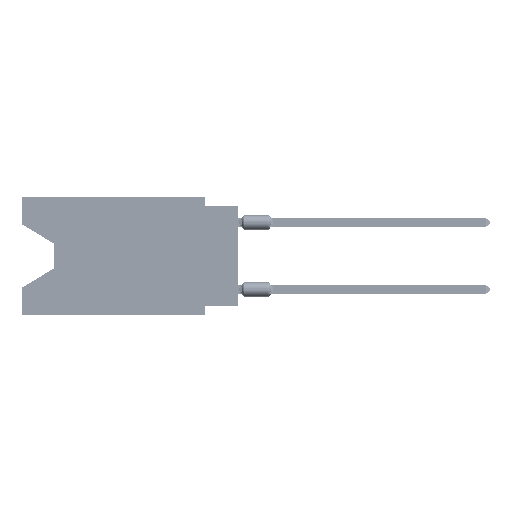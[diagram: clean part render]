
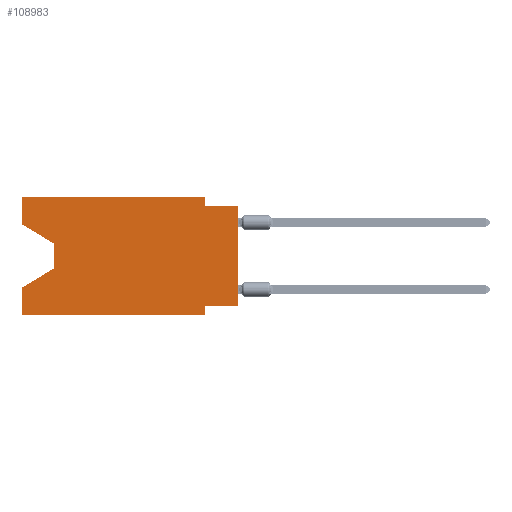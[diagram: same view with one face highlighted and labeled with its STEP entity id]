
A CAD part, left-side view. The second image highlights one B-rep face of the part: STEP entity #108983.
In plain terms, the highlighted planar face has unit normal (-1, 0, 0).
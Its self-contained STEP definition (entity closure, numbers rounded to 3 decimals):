
#1563 = LINE ( 'NONE', #73223, #68733 ) ;
#3938 = VECTOR ( 'NONE', #65482, 1000. ) ;
#7333 = EDGE_CURVE ( 'NONE', #61866, #8219, #95797, .T. ) ;
#8219 = VERTEX_POINT ( 'NONE', #72458 ) ;
#8479 = CARTESIAN_POINT ( 'NONE',  ( 0., 16.383, 0. ) ) ;
#8603 = EDGE_LOOP ( 'NONE', ( #39001, #33583, #102089, #32563, #18057, #45045, #89609, #26927, #80280, #47833, #34997, #63965 ) ) ;
#10073 = DIRECTION ( 'NONE',  ( 0., -1., 0. ) ) ;
#13409 = CARTESIAN_POINT ( 'NONE',  ( 0., 2.54, -0.635 ) ) ;
#13628 = CARTESIAN_POINT ( 'NONE',  ( 0., 16.383, -8.89 ) ) ;
#14525 = PLANE ( 'NONE',  #99285 ) ;
#14832 = EDGE_CURVE ( 'NONE', #24774, #77358, #98203, .T. ) ;
#15952 = CARTESIAN_POINT ( 'NONE',  ( 0., 2.54, -8.89 ) ) ;
#17827 = DIRECTION ( 'NONE',  ( 0., 0., 1. ) ) ;
#18057 = ORIENTED_EDGE ( 'NONE', *, *, #14832, .T. ) ;
#21929 = CARTESIAN_POINT ( 'NONE',  ( 0., 16.383, -8.89 ) ) ;
#23082 = DIRECTION ( 'NONE',  ( 0., 0., -1. ) ) ;
#23469 = CARTESIAN_POINT ( 'NONE',  ( 0., 16.383, -6.852 ) ) ;
#24774 = VERTEX_POINT ( 'NONE', #13628 ) ;
#26149 = EDGE_CURVE ( 'NONE', #36776, #42755, #43752, .T. ) ;
#26927 = ORIENTED_EDGE ( 'NONE', *, *, #7333, .T. ) ;
#27738 = VECTOR ( 'NONE', #79029, 1000. ) ;
#29174 = LINE ( 'NONE', #31449, #50981 ) ;
#29979 = VERTEX_POINT ( 'NONE', #8479 ) ;
#30757 = LINE ( 'NONE', #75685, #3938 ) ;
#31062 = DIRECTION ( 'NONE',  ( 1., 0., 0. ) ) ;
#31449 = CARTESIAN_POINT ( 'NONE',  ( 0., 0., -0.635 ) ) ;
#32563 = ORIENTED_EDGE ( 'NONE', *, *, #83424, .F. ) ;
#33583 = ORIENTED_EDGE ( 'NONE', *, *, #49696, .T. ) ;
#34997 = ORIENTED_EDGE ( 'NONE', *, *, #64373, .F. ) ;
#36776 = VERTEX_POINT ( 'NONE', #105055 ) ;
#37343 = EDGE_CURVE ( 'NONE', #108525, #8219, #29174, .T. ) ;
#38431 = LINE ( 'NONE', #107289, #50976 ) ;
#39001 = ORIENTED_EDGE ( 'NONE', *, *, #42190, .T. ) ;
#40830 = VECTOR ( 'NONE', #99917, 1000. ) ;
#41528 = VERTEX_POINT ( 'NONE', #69510 ) ;
#41853 = CARTESIAN_POINT ( 'NONE',  ( 0., 16.383, 0. ) ) ;
#42190 = EDGE_CURVE ( 'NONE', #54422, #41528, #38431, .T. ) ;
#42755 = VERTEX_POINT ( 'NONE', #23469 ) ;
#42759 = VECTOR ( 'NONE', #17827, 1000. ) ;
#42894 = LINE ( 'NONE', #77593, #108500 ) ;
#43752 = LINE ( 'NONE', #111505, #27738 ) ;
#45045 = ORIENTED_EDGE ( 'NONE', *, *, #63858, .F. ) ;
#47524 = DIRECTION ( 'NONE',  ( 0., -0.855, -0.519 ) ) ;
#47833 = ORIENTED_EDGE ( 'NONE', *, *, #98947, .F. ) ;
#49696 = EDGE_CURVE ( 'NONE', #41528, #36776, #42894, .T. ) ;
#49934 = CARTESIAN_POINT ( 'NONE',  ( 0., 16.383, 0. ) ) ;
#50976 = VECTOR ( 'NONE', #47524, 1000. ) ;
#50981 = VECTOR ( 'NONE', #55368, 1000. ) ;
#53340 = CARTESIAN_POINT ( 'NONE',  ( 0., 16.383, 0. ) ) ;
#54422 = VERTEX_POINT ( 'NONE', #73535 ) ;
#55368 = DIRECTION ( 'NONE',  ( 0., -1., 0. ) ) ;
#60195 = LINE ( 'NONE', #53340, #109395 ) ;
#61063 = DIRECTION ( 'NONE',  ( 0., 0., -1. ) ) ;
#61866 = VERTEX_POINT ( 'NONE', #100586 ) ;
#62701 = CARTESIAN_POINT ( 'NONE',  ( 0., 2.54, 0. ) ) ;
#63858 = EDGE_CURVE ( 'NONE', #101063, #77358, #76287, .T. ) ;
#63910 = VECTOR ( 'NONE', #66632, 1000. ) ;
#63965 = ORIENTED_EDGE ( 'NONE', *, *, #96298, .F. ) ;
#64373 = EDGE_CURVE ( 'NONE', #29979, #87907, #60195, .T. ) ;
#65482 = DIRECTION ( 'NONE',  ( 0., 0., -1. ) ) ;
#66632 = DIRECTION ( 'NONE',  ( 0., 0., -1. ) ) ;
#68375 = CARTESIAN_POINT ( 'NONE',  ( 0., 2.54, -8.89 ) ) ;
#68538 = CARTESIAN_POINT ( 'NONE',  ( 0., 0., 0. ) ) ;
#68733 = VECTOR ( 'NONE', #99409, 1000. ) ;
#69510 = CARTESIAN_POINT ( 'NONE',  ( 0., 13.97, -3.505 ) ) ;
#72458 = CARTESIAN_POINT ( 'NONE',  ( 0., 0., -0.635 ) ) ;
#73223 = CARTESIAN_POINT ( 'NONE',  ( 0., 16.383, 0. ) ) ;
#73535 = CARTESIAN_POINT ( 'NONE',  ( 0., 16.383, -2.038 ) ) ;
#73833 = EDGE_CURVE ( 'NONE', #61866, #101063, #78350, .T. ) ;
#73884 = DIRECTION ( 'NONE',  ( 0., 0., 1. ) ) ;
#74381 = VECTOR ( 'NONE', #73884, 1000. ) ;
#75685 = CARTESIAN_POINT ( 'NONE',  ( 0., 2.54, 0. ) ) ;
#76287 = LINE ( 'NONE', #15952, #63910 ) ;
#77358 = VERTEX_POINT ( 'NONE', #68375 ) ;
#77593 = CARTESIAN_POINT ( 'NONE',  ( 0., 13.97, -3.505 ) ) ;
#78350 = LINE ( 'NONE', #87447, #40830 ) ;
#79029 = DIRECTION ( 'NONE',  ( 0., 0.855, -0.519 ) ) ;
#80280 = ORIENTED_EDGE ( 'NONE', *, *, #37343, .F. ) ;
#81181 = VECTOR ( 'NONE', #91349, 1000. ) ;
#83424 = EDGE_CURVE ( 'NONE', #24774, #42755, #1563, .T. ) ;
#84663 = LINE ( 'NONE', #49934, #74381 ) ;
#87447 = CARTESIAN_POINT ( 'NONE',  ( 0., 0., -8.255 ) ) ;
#87907 = VERTEX_POINT ( 'NONE', #62701 ) ;
#89609 = ORIENTED_EDGE ( 'NONE', *, *, #73833, .F. ) ;
#91349 = DIRECTION ( 'NONE',  ( 0., -1., 0. ) ) ;
#95797 = LINE ( 'NONE', #68538, #42759 ) ;
#96298 = EDGE_CURVE ( 'NONE', #54422, #29979, #84663, .T. ) ;
#98203 = LINE ( 'NONE', #21929, #81181 ) ;
#98947 = EDGE_CURVE ( 'NONE', #87907, #108525, #30757, .T. ) ;
#99285 = AXIS2_PLACEMENT_3D ( 'NONE', #41853, #31062, #23082 ) ;
#99409 = DIRECTION ( 'NONE',  ( 0., 0., 1. ) ) ;
#99917 = DIRECTION ( 'NONE',  ( 0., 1., 0. ) ) ;
#100586 = CARTESIAN_POINT ( 'NONE',  ( 0., 0., -8.255 ) ) ;
#101063 = VERTEX_POINT ( 'NONE', #102566 ) ;
#102089 = ORIENTED_EDGE ( 'NONE', *, *, #26149, .T. ) ;
#102566 = CARTESIAN_POINT ( 'NONE',  ( 0., 2.54, -8.255 ) ) ;
#105055 = CARTESIAN_POINT ( 'NONE',  ( 0., 13.97, -5.385 ) ) ;
#107289 = CARTESIAN_POINT ( 'NONE',  ( 0., 16.383, -2.038 ) ) ;
#108500 = VECTOR ( 'NONE', #61063, 1000. ) ;
#108525 = VERTEX_POINT ( 'NONE', #13409 ) ;
#108983 = ADVANCED_FACE ( 'NONE', ( #110693 ), #14525, .F. ) ;
#109395 = VECTOR ( 'NONE', #10073, 1000. ) ;
#110693 = FACE_OUTER_BOUND ( 'NONE', #8603, .T. ) ;
#111505 = CARTESIAN_POINT ( 'NONE',  ( 0., 13.97, -5.385 ) ) ;
